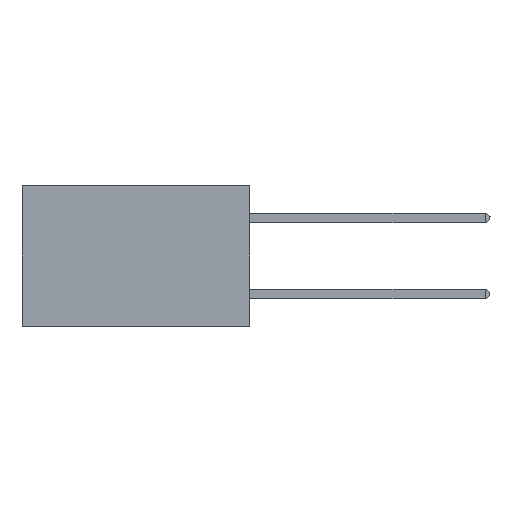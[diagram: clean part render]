
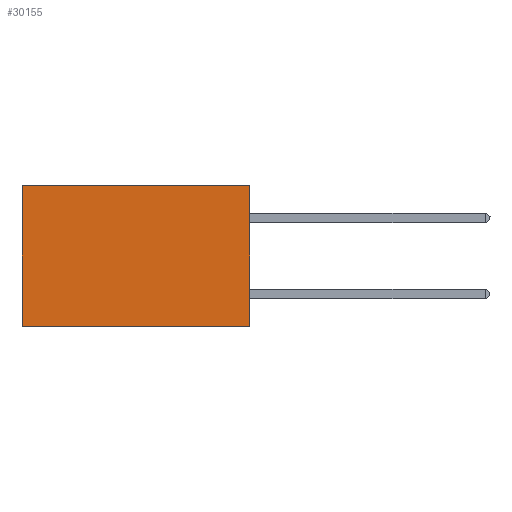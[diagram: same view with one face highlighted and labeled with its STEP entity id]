
A CAD part, left-side view. The second image highlights one B-rep face of the part: STEP entity #30155.
In plain terms, the highlighted planar face has unit normal (-1, 0, 0).
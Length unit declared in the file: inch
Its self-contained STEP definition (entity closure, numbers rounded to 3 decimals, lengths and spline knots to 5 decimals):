
#105 = CARTESIAN_POINT ( 'NONE',  ( 0.2875, 0., 0. ) ) ;
#228 = CARTESIAN_POINT ( 'NONE',  ( 0.2875, 0.6, -0.37 ) ) ;
#1226 = CARTESIAN_POINT ( 'NONE',  ( 0.2875, 0., 0. ) ) ;
#2516 = LINE ( 'NONE', #105, #29139 ) ;
#2844 = CARTESIAN_POINT ( 'NONE',  ( 0.2875, 0., 0. ) ) ;
#3129 = ORIENTED_EDGE ( 'NONE', *, *, #33128, .T. ) ;
#3698 = VECTOR ( 'NONE', #12425, 39.37008 ) ;
#4408 = VERTEX_POINT ( 'NONE', #2844 ) ;
#5425 = VECTOR ( 'NONE', #16149, 39.37008 ) ;
#6133 = EDGE_CURVE ( 'NONE', #10307, #9471, #16634, .T. ) ;
#7236 = LINE ( 'NONE', #1226, #32068 ) ;
#8437 = CARTESIAN_POINT ( 'NONE',  ( 0.2875, 0., -0.37 ) ) ;
#9471 = VERTEX_POINT ( 'NONE', #228 ) ;
#10307 = VERTEX_POINT ( 'NONE', #8437 ) ;
#10579 = VERTEX_POINT ( 'NONE', #13980 ) ;
#10594 = PLANE ( 'NONE',  #19577 ) ;
#12425 = DIRECTION ( 'NONE',  ( 0., 1., 0. ) ) ;
#12467 = EDGE_CURVE ( 'NONE', #10579, #9471, #18300, .T. ) ;
#13156 = DIRECTION ( 'NONE',  ( 1., 0., 0. ) ) ;
#13881 = EDGE_CURVE ( 'NONE', #4408, #10307, #7236, .T. ) ;
#13980 = CARTESIAN_POINT ( 'NONE',  ( 0.2875, 0.6, 0. ) ) ;
#14809 = EDGE_LOOP ( 'NONE', ( #31012, #21514, #24149, #3129 ) ) ;
#16149 = DIRECTION ( 'NONE',  ( 0., 0., -1. ) ) ;
#16634 = LINE ( 'NONE', #25199, #3698 ) ;
#18237 = DIRECTION ( 'NONE',  ( 0., 1., 0. ) ) ;
#18300 = LINE ( 'NONE', #28949, #5425 ) ;
#19577 = AXIS2_PLACEMENT_3D ( 'NONE', #28542, #13156, #31079 ) ;
#21514 = ORIENTED_EDGE ( 'NONE', *, *, #6133, .F. ) ;
#24149 = ORIENTED_EDGE ( 'NONE', *, *, #13881, .F. ) ;
#25199 = CARTESIAN_POINT ( 'NONE',  ( 0.2875, 0., -0.37 ) ) ;
#25950 = FACE_OUTER_BOUND ( 'NONE', #14809, .T. ) ;
#26980 = DIRECTION ( 'NONE',  ( 0., 0., -1. ) ) ;
#28542 = CARTESIAN_POINT ( 'NONE',  ( 0.2875, 0., 0. ) ) ;
#28949 = CARTESIAN_POINT ( 'NONE',  ( 0.2875, 0.6, 0. ) ) ;
#29139 = VECTOR ( 'NONE', #18237, 39.37008 ) ;
#30155 = ADVANCED_FACE ( 'NONE', ( #25950 ), #10594, .F. ) ;
#31012 = ORIENTED_EDGE ( 'NONE', *, *, #12467, .T. ) ;
#31079 = DIRECTION ( 'NONE',  ( 0., 0., -1. ) ) ;
#32068 = VECTOR ( 'NONE', #26980, 39.37008 ) ;
#33128 = EDGE_CURVE ( 'NONE', #4408, #10579, #2516, .T. ) ;
